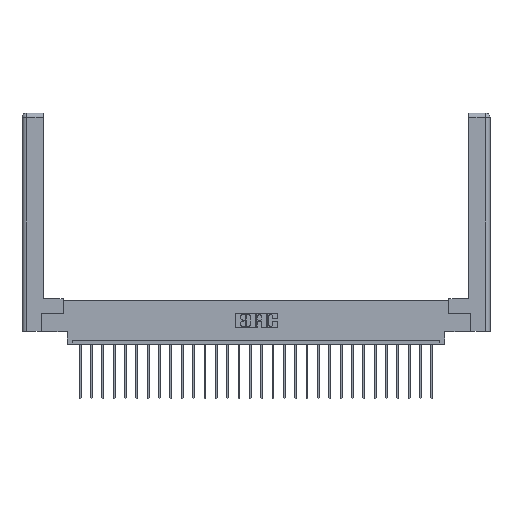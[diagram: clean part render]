
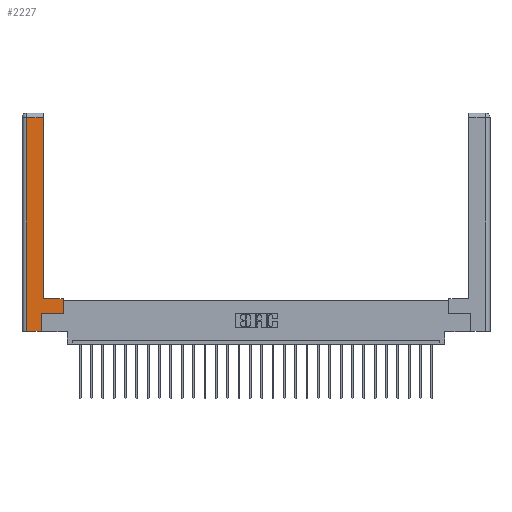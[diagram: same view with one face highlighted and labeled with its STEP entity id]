
A CAD part, top view. The second image highlights one B-rep face of the part: STEP entity #2227.
In plain terms, the highlighted planar face has unit normal (0, 0, 1).
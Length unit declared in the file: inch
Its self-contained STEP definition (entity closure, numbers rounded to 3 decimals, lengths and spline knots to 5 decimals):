
#183 = EDGE_CURVE ( 'NONE', #11775, #339, #1350, .T. ) ;
#339 = VERTEX_POINT ( 'NONE', #9084 ) ;
#449 = VECTOR ( 'NONE', #27130, 39.37008 ) ;
#649 = ORIENTED_EDGE ( 'NONE', *, *, #11013, .T. ) ;
#1350 = LINE ( 'NONE', #18921, #10100 ) ;
#1891 = CARTESIAN_POINT ( 'NONE',  ( 0., 0., 0. ) ) ;
#2134 = VECTOR ( 'NONE', #25334, 39.37008 ) ;
#2227 = ADVANCED_FACE ( 'NONE', ( #15319 ), #8396, .F. ) ;
#2476 = VECTOR ( 'NONE', #5272, 39.37008 ) ;
#2478 = LINE ( 'NONE', #12730, #11866 ) ;
#2722 = CARTESIAN_POINT ( 'NONE',  ( 0.295, 2.94, 0. ) ) ;
#3200 = ORIENTED_EDGE ( 'NONE', *, *, #23483, .T. ) ;
#3315 = VECTOR ( 'NONE', #9395, 39.37008 ) ;
#4072 = DIRECTION ( 'NONE',  ( 0., 0., -1. ) ) ;
#5087 = ORIENTED_EDGE ( 'NONE', *, *, #22345, .T. ) ;
#5272 = DIRECTION ( 'NONE',  ( -1., 0., 0. ) ) ;
#5543 = DIRECTION ( 'NONE',  ( -1., 0., 0. ) ) ;
#5831 = CARTESIAN_POINT ( 'NONE',  ( 0.565, 0.45, 0. ) ) ;
#6723 = LINE ( 'NONE', #8029, #10388 ) ;
#7110 = ORIENTED_EDGE ( 'NONE', *, *, #183, .T. ) ;
#7330 = CARTESIAN_POINT ( 'NONE',  ( 0.295, 0.45, 0. ) ) ;
#7634 = VERTEX_POINT ( 'NONE', #11788 ) ;
#7715 = EDGE_CURVE ( 'NONE', #23039, #11775, #18609, .T. ) ;
#8029 = CARTESIAN_POINT ( 'NONE',  ( 0.295, 3., 0. ) ) ;
#8396 = PLANE ( 'NONE',  #19371 ) ;
#8402 = DIRECTION ( 'NONE',  ( 0., 1., 0. ) ) ;
#8540 = LINE ( 'NONE', #5831, #2134 ) ;
#9084 = CARTESIAN_POINT ( 'NONE',  ( 0.265, 0., 0. ) ) ;
#9395 = DIRECTION ( 'NONE',  ( 1., 0., 0. ) ) ;
#9667 = CARTESIAN_POINT ( 'NONE',  ( 0.565, 0.245, 0. ) ) ;
#9695 = VERTEX_POINT ( 'NONE', #2722 ) ;
#10016 = CARTESIAN_POINT ( 'NONE',  ( 0.0615, 0., 0. ) ) ;
#10100 = VECTOR ( 'NONE', #25418, 39.37008 ) ;
#10388 = VECTOR ( 'NONE', #8402, 39.37008 ) ;
#11013 = EDGE_CURVE ( 'NONE', #11331, #7634, #16907, .T. ) ;
#11076 = CARTESIAN_POINT ( 'NONE',  ( 0.0615, 0., 0. ) ) ;
#11331 = VERTEX_POINT ( 'NONE', #24441 ) ;
#11775 = VERTEX_POINT ( 'NONE', #11076 ) ;
#11788 = CARTESIAN_POINT ( 'NONE',  ( 0.295, 0.45, 0. ) ) ;
#11866 = VECTOR ( 'NONE', #25511, 39.37008 ) ;
#12061 = ORIENTED_EDGE ( 'NONE', *, *, #7715, .T. ) ;
#12730 = CARTESIAN_POINT ( 'NONE',  ( 0.265, 0.245, 0. ) ) ;
#13209 = VERTEX_POINT ( 'NONE', #17504 ) ;
#13723 = LINE ( 'NONE', #9667, #3315 ) ;
#15319 = FACE_OUTER_BOUND ( 'NONE', #18480, .T. ) ;
#15854 = CARTESIAN_POINT ( 'NONE',  ( 0.0615, 2.94, 0. ) ) ;
#16048 = ORIENTED_EDGE ( 'NONE', *, *, #16338, .T. ) ;
#16338 = EDGE_CURVE ( 'NONE', #339, #25326, #2478, .T. ) ;
#16907 = LINE ( 'NONE', #7330, #2476 ) ;
#17504 = CARTESIAN_POINT ( 'NONE',  ( 0.565, 0.245, 0. ) ) ;
#18480 = EDGE_LOOP ( 'NONE', ( #25440, #18910, #12061, #7110, #16048, #3200, #5087, #649 ) ) ;
#18501 = EDGE_CURVE ( 'NONE', #7634, #9695, #6723, .T. ) ;
#18586 = CARTESIAN_POINT ( 'NONE',  ( 0.0615, 2.94, 0. ) ) ;
#18609 = LINE ( 'NONE', #10016, #449 ) ;
#18910 = ORIENTED_EDGE ( 'NONE', *, *, #21496, .T. ) ;
#18921 = CARTESIAN_POINT ( 'NONE',  ( 0.265, 0., 0. ) ) ;
#19371 = AXIS2_PLACEMENT_3D ( 'NONE', #1891, #4072, #25096 ) ;
#19661 = LINE ( 'NONE', #18586, #24698 ) ;
#21011 = CARTESIAN_POINT ( 'NONE',  ( 0.265, 0.245, 0. ) ) ;
#21496 = EDGE_CURVE ( 'NONE', #9695, #23039, #19661, .T. ) ;
#22345 = EDGE_CURVE ( 'NONE', #13209, #11331, #8540, .T. ) ;
#23039 = VERTEX_POINT ( 'NONE', #15854 ) ;
#23483 = EDGE_CURVE ( 'NONE', #25326, #13209, #13723, .T. ) ;
#24441 = CARTESIAN_POINT ( 'NONE',  ( 0.565, 0.45, 0. ) ) ;
#24698 = VECTOR ( 'NONE', #5543, 39.37008 ) ;
#25096 = DIRECTION ( 'NONE',  ( -1., 0., 0. ) ) ;
#25326 = VERTEX_POINT ( 'NONE', #21011 ) ;
#25334 = DIRECTION ( 'NONE',  ( 0., 1., 0. ) ) ;
#25418 = DIRECTION ( 'NONE',  ( 1., 0., 0. ) ) ;
#25440 = ORIENTED_EDGE ( 'NONE', *, *, #18501, .T. ) ;
#25511 = DIRECTION ( 'NONE',  ( 0., 1., 0. ) ) ;
#27130 = DIRECTION ( 'NONE',  ( 0., -1., 0. ) ) ;
